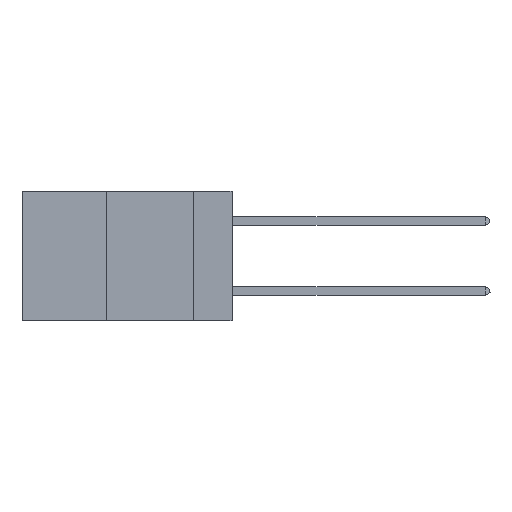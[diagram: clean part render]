
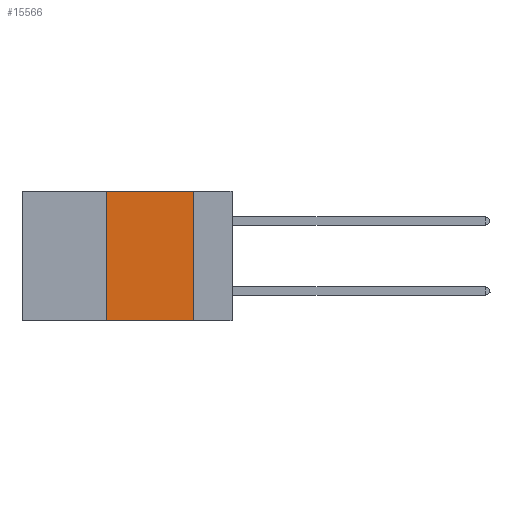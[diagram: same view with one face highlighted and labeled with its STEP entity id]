
A CAD part, left-side view. The second image highlights one B-rep face of the part: STEP entity #15566.
In plain terms, the highlighted planar face has unit normal (-1, 0, 0).
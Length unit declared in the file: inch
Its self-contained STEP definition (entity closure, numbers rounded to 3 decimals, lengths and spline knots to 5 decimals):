
#115 = EDGE_CURVE ( 'NONE', #1073, #5523, #13907, .T. ) ;
#1073 = VERTEX_POINT ( 'NONE', #2315 ) ;
#1308 = LINE ( 'NONE', #15551, #18810 ) ;
#1481 = EDGE_LOOP ( 'NONE', ( #2446, #4253, #11104, #7398 ) ) ;
#2315 = CARTESIAN_POINT ( 'NONE',  ( 0., 0.36, -0.37 ) ) ;
#2352 = VECTOR ( 'NONE', #12977, 39.37008 ) ;
#2446 = ORIENTED_EDGE ( 'NONE', *, *, #14173, .F. ) ;
#2832 = VERTEX_POINT ( 'NONE', #4504 ) ;
#4253 = ORIENTED_EDGE ( 'NONE', *, *, #14947, .F. ) ;
#4504 = CARTESIAN_POINT ( 'NONE',  ( 0., 0.36, 0. ) ) ;
#5425 = CARTESIAN_POINT ( 'NONE',  ( 0., 0.11, 0. ) ) ;
#5478 = DIRECTION ( 'NONE',  ( 0., 0., 1. ) ) ;
#5523 = VERTEX_POINT ( 'NONE', #11109 ) ;
#5922 = LINE ( 'NONE', #14540, #6147 ) ;
#6147 = VECTOR ( 'NONE', #8887, 39.37008 ) ;
#6214 = CARTESIAN_POINT ( 'NONE',  ( 0., 0.6, 0. ) ) ;
#6249 = CARTESIAN_POINT ( 'NONE',  ( 0., 0.11, 0. ) ) ;
#6341 = DIRECTION ( 'NONE',  ( 0., 0., -1. ) ) ;
#6524 = DIRECTION ( 'NONE',  ( 0., -1., 0. ) ) ;
#7398 = ORIENTED_EDGE ( 'NONE', *, *, #115, .T. ) ;
#8887 = DIRECTION ( 'NONE',  ( 0., -1., 0. ) ) ;
#8980 = DIRECTION ( 'NONE',  ( 1., 0., 0. ) ) ;
#9674 = VERTEX_POINT ( 'NONE', #6249 ) ;
#9999 = LINE ( 'NONE', #5425, #2352 ) ;
#10631 = FACE_OUTER_BOUND ( 'NONE', #1481, .T. ) ;
#11104 = ORIENTED_EDGE ( 'NONE', *, *, #11489, .F. ) ;
#11109 = CARTESIAN_POINT ( 'NONE',  ( 0., 0.11, -0.37 ) ) ;
#11489 = EDGE_CURVE ( 'NONE', #1073, #2832, #1308, .T. ) ;
#12066 = PLANE ( 'NONE',  #17853 ) ;
#12977 = DIRECTION ( 'NONE',  ( 0., 0., -1. ) ) ;
#13907 = LINE ( 'NONE', #14940, #15281 ) ;
#14173 = EDGE_CURVE ( 'NONE', #9674, #5523, #9999, .T. ) ;
#14540 = CARTESIAN_POINT ( 'NONE',  ( 0., 0.6, 0. ) ) ;
#14940 = CARTESIAN_POINT ( 'NONE',  ( 0., 0.6, -0.37 ) ) ;
#14947 = EDGE_CURVE ( 'NONE', #2832, #9674, #5922, .T. ) ;
#15281 = VECTOR ( 'NONE', #6524, 39.37008 ) ;
#15551 = CARTESIAN_POINT ( 'NONE',  ( 0., 0.36, 0. ) ) ;
#15566 = ADVANCED_FACE ( 'NONE', ( #10631 ), #12066, .F. ) ;
#17853 = AXIS2_PLACEMENT_3D ( 'NONE', #6214, #8980, #6341 ) ;
#18810 = VECTOR ( 'NONE', #5478, 39.37008 ) ;
